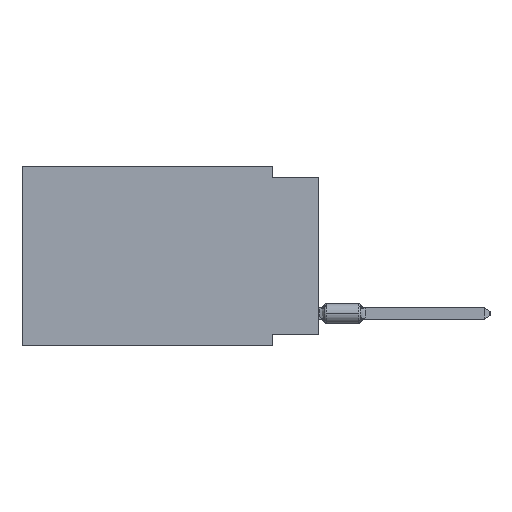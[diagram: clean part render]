
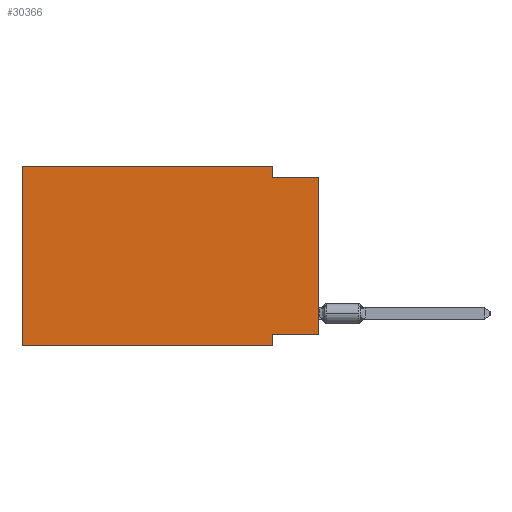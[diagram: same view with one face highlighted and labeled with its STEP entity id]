
A CAD part, left-side view. The second image highlights one B-rep face of the part: STEP entity #30366.
In plain terms, the highlighted planar face has unit normal (-1, 0, 0).
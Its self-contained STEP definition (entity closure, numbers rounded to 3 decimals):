
#26 = LINE ( 'NONE', #3618, #8004 ) ;
#194 = VECTOR ( 'NONE', #12850, 1000. ) ;
#1319 = CARTESIAN_POINT ( 'NONE',  ( 0., 0., -9.271 ) ) ;
#2409 = ORIENTED_EDGE ( 'NONE', *, *, #22897, .F. ) ;
#3618 = CARTESIAN_POINT ( 'NONE',  ( 0., 0., 0. ) ) ;
#4829 = FACE_OUTER_BOUND ( 'NONE', #20374, .T. ) ;
#5643 = EDGE_CURVE ( 'NONE', #29076, #25987, #28739, .T. ) ;
#5876 = VECTOR ( 'NONE', #6396, 1000. ) ;
#6041 = CARTESIAN_POINT ( 'NONE',  ( 0., 16.383, 0. ) ) ;
#6389 = DIRECTION ( 'NONE',  ( 0., 0., -1. ) ) ;
#6396 = DIRECTION ( 'NONE',  ( 0., -1., 0. ) ) ;
#7295 = CARTESIAN_POINT ( 'NONE',  ( 0., 2.54, -0.635 ) ) ;
#7621 = VERTEX_POINT ( 'NONE', #37703 ) ;
#8004 = VECTOR ( 'NONE', #14138, 1000. ) ;
#8865 = CARTESIAN_POINT ( 'NONE',  ( 0., 2.54, -9.906 ) ) ;
#9843 = VERTEX_POINT ( 'NONE', #21208 ) ;
#10117 = ORIENTED_EDGE ( 'NONE', *, *, #30147, .F. ) ;
#10989 = CARTESIAN_POINT ( 'NONE',  ( 0., 0., -0.635 ) ) ;
#12237 = DIRECTION ( 'NONE',  ( 1., 0., 0. ) ) ;
#12850 = DIRECTION ( 'NONE',  ( 0., -1., 0. ) ) ;
#13162 = ORIENTED_EDGE ( 'NONE', *, *, #27999, .F. ) ;
#13874 = ORIENTED_EDGE ( 'NONE', *, *, #20834, .T. ) ;
#14138 = DIRECTION ( 'NONE',  ( 0., 0., 1. ) ) ;
#14990 = DIRECTION ( 'NONE',  ( 0., 1., 0. ) ) ;
#15293 = DIRECTION ( 'NONE',  ( 0., 0., -1. ) ) ;
#15905 = LINE ( 'NONE', #6041, #16470 ) ;
#16470 = VECTOR ( 'NONE', #43425, 1000. ) ;
#16768 = VECTOR ( 'NONE', #6389, 1000. ) ;
#19464 = EDGE_CURVE ( 'NONE', #9843, #41733, #35950, .T. ) ;
#19484 = AXIS2_PLACEMENT_3D ( 'NONE', #35729, #12237, #39298 ) ;
#19955 = VERTEX_POINT ( 'NONE', #40422 ) ;
#20002 = LINE ( 'NONE', #26936, #194 ) ;
#20096 = LINE ( 'NONE', #20315, #33739 ) ;
#20315 = CARTESIAN_POINT ( 'NONE',  ( 0., 0., -0.635 ) ) ;
#20374 = EDGE_LOOP ( 'NONE', ( #13874, #10117, #39591, #2409, #13162, #22350, #22143, #26403 ) ) ;
#20834 = EDGE_CURVE ( 'NONE', #19955, #37918, #26, .T. ) ;
#21208 = CARTESIAN_POINT ( 'NONE',  ( 0., 2.54, -9.271 ) ) ;
#22143 = ORIENTED_EDGE ( 'NONE', *, *, #19464, .F. ) ;
#22350 = ORIENTED_EDGE ( 'NONE', *, *, #23352, .T. ) ;
#22897 = EDGE_CURVE ( 'NONE', #7621, #29076, #27453, .T. ) ;
#23352 = EDGE_CURVE ( 'NONE', #35699, #41733, #20002, .T. ) ;
#25987 = VERTEX_POINT ( 'NONE', #7295 ) ;
#26403 = ORIENTED_EDGE ( 'NONE', *, *, #26939, .F. ) ;
#26936 = CARTESIAN_POINT ( 'NONE',  ( 0., 16.383, -9.906 ) ) ;
#26939 = EDGE_CURVE ( 'NONE', #19955, #9843, #34917, .T. ) ;
#27453 = LINE ( 'NONE', #37278, #5876 ) ;
#27999 = EDGE_CURVE ( 'NONE', #35699, #7621, #15905, .T. ) ;
#28739 = LINE ( 'NONE', #39227, #42689 ) ;
#28806 = PLANE ( 'NONE',  #19484 ) ;
#29076 = VERTEX_POINT ( 'NONE', #40183 ) ;
#30147 = EDGE_CURVE ( 'NONE', #25987, #37918, #20096, .T. ) ;
#30366 = ADVANCED_FACE ( 'NONE', ( #4829 ), #28806, .F. ) ;
#33739 = VECTOR ( 'NONE', #33955, 1000. ) ;
#33955 = DIRECTION ( 'NONE',  ( 0., -1., 0. ) ) ;
#34917 = LINE ( 'NONE', #1319, #42224 ) ;
#35699 = VERTEX_POINT ( 'NONE', #37395 ) ;
#35729 = CARTESIAN_POINT ( 'NONE',  ( 0., 16.383, 0. ) ) ;
#35950 = LINE ( 'NONE', #8865, #16768 ) ;
#37278 = CARTESIAN_POINT ( 'NONE',  ( 0., 16.383, 0. ) ) ;
#37395 = CARTESIAN_POINT ( 'NONE',  ( 0., 16.383, -9.906 ) ) ;
#37703 = CARTESIAN_POINT ( 'NONE',  ( 0., 16.383, 0. ) ) ;
#37918 = VERTEX_POINT ( 'NONE', #10989 ) ;
#39227 = CARTESIAN_POINT ( 'NONE',  ( 0., 2.54, 0. ) ) ;
#39298 = DIRECTION ( 'NONE',  ( 0., 0., -1. ) ) ;
#39591 = ORIENTED_EDGE ( 'NONE', *, *, #5643, .F. ) ;
#40183 = CARTESIAN_POINT ( 'NONE',  ( 0., 2.54, 0. ) ) ;
#40422 = CARTESIAN_POINT ( 'NONE',  ( 0., 0., -9.271 ) ) ;
#41502 = CARTESIAN_POINT ( 'NONE',  ( 0., 2.54, -9.906 ) ) ;
#41733 = VERTEX_POINT ( 'NONE', #41502 ) ;
#42224 = VECTOR ( 'NONE', #14990, 1000. ) ;
#42689 = VECTOR ( 'NONE', #15293, 1000. ) ;
#43425 = DIRECTION ( 'NONE',  ( 0., 0., 1. ) ) ;
